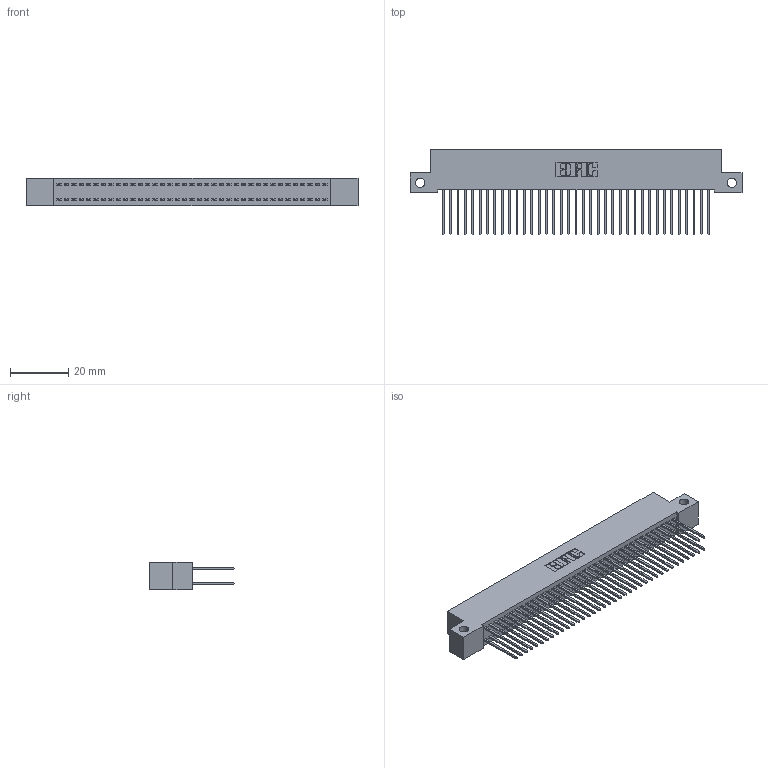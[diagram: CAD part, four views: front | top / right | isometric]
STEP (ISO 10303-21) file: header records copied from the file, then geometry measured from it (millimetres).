
FILE_DESCRIPTION (( 'STEP AP203' ), '1' );
FILE_NAME ('342-074-540-212.STEP', '2018-08-13T11:23:27', ( '' ), ( '' ), 'SwSTEP 2.0', 'SolidWorks 2016', '' );
FILE_SCHEMA (( 'CONFIG_CONTROL_DESIGN' ));
Length unit declared in the file: inch
Products named in the file (3): 342 Part_Side Mount; 345-292-001_345-293-140; 342-074-540-212
Assembly tree (75 placements, depth 2):
  342-074-540-212
    342 Part_Side Mount
    345-292-001_345-293-140  x74
Bounding box: 114.3 x 29.47 x 9.4 mm (x, y, z)
Volume: 10452.8 mm3; surface area: 17978.7 mm2
Topology: 75 solids, 75 shells, 3958 faces, 11769 edges, 7746 vertices
Faces by surface type: plane 2730, cylinder 1228
Entity records: 24339 total; most frequent: CARTESIAN_POINT 4038, ORIENTED_EDGE 3974, DIRECTION 3459, EDGE_CURVE 1987, LINE 1859, VECTOR 1859, VERTEX_POINT 1322, AXIS2_PLACEMENT_3D 800
